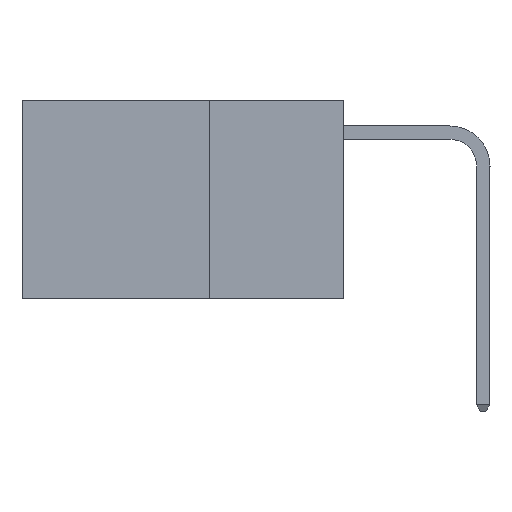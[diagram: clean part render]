
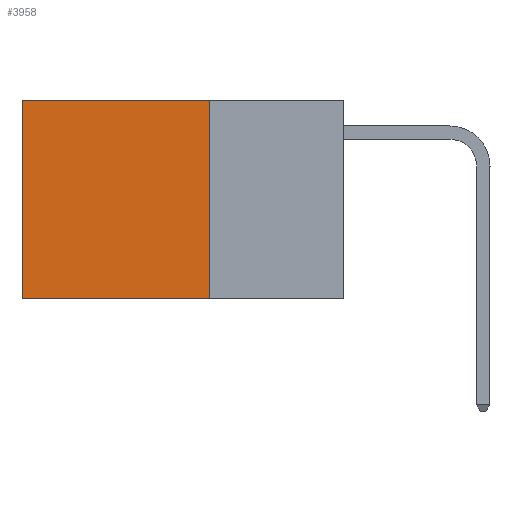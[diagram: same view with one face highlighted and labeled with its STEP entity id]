
A CAD part, left-side view. The second image highlights one B-rep face of the part: STEP entity #3958.
In plain terms, the highlighted planar face has unit normal (-1, 0, 0).
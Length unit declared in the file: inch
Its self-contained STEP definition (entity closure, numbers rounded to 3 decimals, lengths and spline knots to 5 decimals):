
#282 = VECTOR ( 'NONE', #28296, 39.37008 ) ;
#602 = LINE ( 'NONE', #23717, #282 ) ;
#3958 = ADVANCED_FACE ( 'NONE', ( #10102 ), #8682, .F. ) ;
#4090 = DIRECTION ( 'NONE',  ( 0., 0., -1. ) ) ;
#4208 = CARTESIAN_POINT ( 'NONE',  ( 0.2625, 0.25, 0. ) ) ;
#4502 = ORIENTED_EDGE ( 'NONE', *, *, #19044, .T. ) ;
#5322 = LINE ( 'NONE', #4208, #10791 ) ;
#6559 = CARTESIAN_POINT ( 'NONE',  ( 0.2625, 0.6, 0. ) ) ;
#6590 = DIRECTION ( 'NONE',  ( 0., 0., -1. ) ) ;
#7630 = ORIENTED_EDGE ( 'NONE', *, *, #18267, .T. ) ;
#8409 = EDGE_LOOP ( 'NONE', ( #4502, #19139, #11681, #7630 ) ) ;
#8682 = PLANE ( 'NONE',  #23640 ) ;
#9865 = LINE ( 'NONE', #20560, #22279 ) ;
#10102 = FACE_OUTER_BOUND ( 'NONE', #8409, .T. ) ;
#10791 = VECTOR ( 'NONE', #25130, 39.37008 ) ;
#11681 = ORIENTED_EDGE ( 'NONE', *, *, #21129, .F. ) ;
#11830 = VECTOR ( 'NONE', #26611, 39.37008 ) ;
#12952 = VERTEX_POINT ( 'NONE', #20788 ) ;
#13358 = CARTESIAN_POINT ( 'NONE',  ( 0.2625, 0.25, 0. ) ) ;
#14981 = EDGE_CURVE ( 'NONE', #23877, #12952, #602, .T. ) ;
#18052 = DIRECTION ( 'NONE',  ( 1., 0., 0. ) ) ;
#18267 = EDGE_CURVE ( 'NONE', #27976, #28286, #5322, .T. ) ;
#19044 = EDGE_CURVE ( 'NONE', #28286, #12952, #26339, .T. ) ;
#19139 = ORIENTED_EDGE ( 'NONE', *, *, #14981, .F. ) ;
#20069 = CARTESIAN_POINT ( 'NONE',  ( 0.2625, 0.25, -0.37 ) ) ;
#20560 = CARTESIAN_POINT ( 'NONE',  ( 0.2625, 0.25, 0. ) ) ;
#20788 = CARTESIAN_POINT ( 'NONE',  ( 0.2625, 0.6, -0.37 ) ) ;
#21129 = EDGE_CURVE ( 'NONE', #27976, #23877, #9865, .T. ) ;
#22279 = VECTOR ( 'NONE', #6590, 39.37008 ) ;
#23640 = AXIS2_PLACEMENT_3D ( 'NONE', #13358, #18052, #4090 ) ;
#23717 = CARTESIAN_POINT ( 'NONE',  ( 0.2625, 0.25, -0.37 ) ) ;
#23877 = VERTEX_POINT ( 'NONE', #20069 ) ;
#25130 = DIRECTION ( 'NONE',  ( 0., 1., 0. ) ) ;
#26339 = LINE ( 'NONE', #29078, #11830 ) ;
#26611 = DIRECTION ( 'NONE',  ( 0., 0., -1. ) ) ;
#27976 = VERTEX_POINT ( 'NONE', #28572 ) ;
#28286 = VERTEX_POINT ( 'NONE', #6559 ) ;
#28296 = DIRECTION ( 'NONE',  ( 0., 1., 0. ) ) ;
#28572 = CARTESIAN_POINT ( 'NONE',  ( 0.2625, 0.25, 0. ) ) ;
#29078 = CARTESIAN_POINT ( 'NONE',  ( 0.2625, 0.6, 0. ) ) ;
